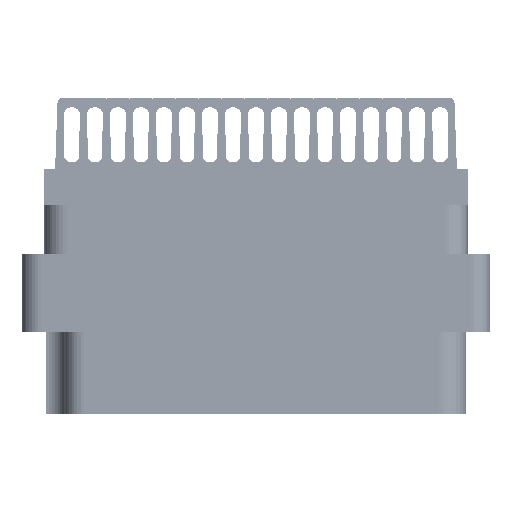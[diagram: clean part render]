
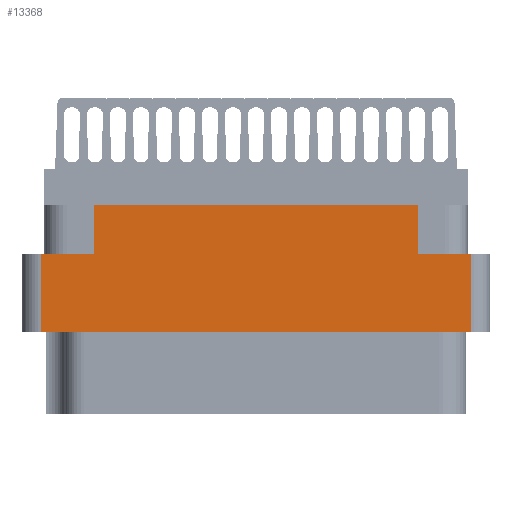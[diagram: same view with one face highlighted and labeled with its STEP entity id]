
A CAD part, left-side view. The second image highlights one B-rep face of the part: STEP entity #13368.
In plain terms, the highlighted planar face has unit normal (-1, 0, 0).
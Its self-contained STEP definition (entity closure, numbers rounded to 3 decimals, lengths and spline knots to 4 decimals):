
#1298 = DIRECTION ( 'NONE',  ( 0., 0., -1. ) ) ;
#3720 = EDGE_CURVE ( 'NONE', #88290, #62367, #60270, .T. ) ;
#4019 = ORIENTED_EDGE ( 'NONE', *, *, #32455, .T. ) ;
#6077 = VECTOR ( 'NONE', #66229, 39.3701 ) ;
#8338 = CARTESIAN_POINT ( 'NONE',  ( -1.375, 0., -0.529 ) ) ;
#9785 = VECTOR ( 'NONE', #70569, 39.3701 ) ;
#10305 = ORIENTED_EDGE ( 'NONE', *, *, #92936, .F. ) ;
#11412 = VERTEX_POINT ( 'NONE', #49687 ) ;
#12026 = VERTEX_POINT ( 'NONE', #71877 ) ;
#12495 = ORIENTED_EDGE ( 'NONE', *, *, #66416, .F. ) ;
#13368 = ADVANCED_FACE ( 'NONE', ( #31602 ), #30020, .T. ) ;
#13901 = VECTOR ( 'NONE', #89599, 39.3701 ) ;
#15624 = DIRECTION ( 'NONE',  ( 0., 1., 0. ) ) ;
#16815 = CARTESIAN_POINT ( 'NONE',  ( -1.375, -0.7005, -0.798 ) ) ;
#18378 = CARTESIAN_POINT ( 'NONE',  ( -1.375, -0.5285, -0.277 ) ) ;
#18799 = VERTEX_POINT ( 'NONE', #53100 ) ;
#23161 = EDGE_LOOP ( 'NONE', ( #43654, #37005, #30594, #29555, #12495, #4019, #10305, #57130 ) ) ;
#26002 = VECTOR ( 'NONE', #35717, 39.3701 ) ;
#26026 = LINE ( 'NONE', #18378, #45294 ) ;
#26498 = CARTESIAN_POINT ( 'NONE',  ( -1.375, 0.5285, -0.277 ) ) ;
#29555 = ORIENTED_EDGE ( 'NONE', *, *, #57769, .T. ) ;
#30020 = PLANE ( 'NONE',  #61913 ) ;
#30327 = CARTESIAN_POINT ( 'NONE',  ( -1.375, 0., -0.277 ) ) ;
#30594 = ORIENTED_EDGE ( 'NONE', *, *, #3720, .F. ) ;
#30751 = CARTESIAN_POINT ( 'NONE',  ( -1.375, 0., -0.277 ) ) ;
#31602 = FACE_OUTER_BOUND ( 'NONE', #23161, .T. ) ;
#32455 = EDGE_CURVE ( 'NONE', #53001, #11412, #26026, .T. ) ;
#34495 = LINE ( 'NONE', #44851, #75499 ) ;
#34787 = CARTESIAN_POINT ( 'NONE',  ( -1.375, 0.7625, -0.117 ) ) ;
#35717 = DIRECTION ( 'NONE',  ( 0., -1., 0. ) ) ;
#37005 = ORIENTED_EDGE ( 'NONE', *, *, #68602, .T. ) ;
#37239 = CARTESIAN_POINT ( 'NONE',  ( -1.375, -0.7625, -0.798 ) ) ;
#37558 = DIRECTION ( 'NONE',  ( -1., 0., 0. ) ) ;
#38107 = VECTOR ( 'NONE', #40411, 39.3701 ) ;
#40411 = DIRECTION ( 'NONE',  ( 0., 0., 1. ) ) ;
#43654 = ORIENTED_EDGE ( 'NONE', *, *, #46906, .F. ) ;
#44851 = CARTESIAN_POINT ( 'NONE',  ( -1.375, 0.7005, -0.798 ) ) ;
#45268 = LINE ( 'NONE', #34787, #26002 ) ;
#45294 = VECTOR ( 'NONE', #84878, 39.3701 ) ;
#46906 = EDGE_CURVE ( 'NONE', #12026, #66844, #60799, .T. ) ;
#48449 = LINE ( 'NONE', #16815, #9785 ) ;
#49687 = CARTESIAN_POINT ( 'NONE',  ( -1.375, -0.5285, -0.117 ) ) ;
#53001 = VERTEX_POINT ( 'NONE', #84582 ) ;
#53100 = CARTESIAN_POINT ( 'NONE',  ( -1.375, 0.5285, -0.117 ) ) ;
#55010 = CARTESIAN_POINT ( 'NONE',  ( -1.375, -0.7005, -0.529 ) ) ;
#57130 = ORIENTED_EDGE ( 'NONE', *, *, #85940, .F. ) ;
#57769 = EDGE_CURVE ( 'NONE', #88290, #93640, #48449, .T. ) ;
#60270 = LINE ( 'NONE', #8338, #73944 ) ;
#60799 = LINE ( 'NONE', #30327, #6077 ) ;
#60881 = LINE ( 'NONE', #26498, #38107 ) ;
#61913 = AXIS2_PLACEMENT_3D ( 'NONE', #37239, #37558, #88225 ) ;
#62367 = VERTEX_POINT ( 'NONE', #72286 ) ;
#66229 = DIRECTION ( 'NONE',  ( 0., -1., 0. ) ) ;
#66416 = EDGE_CURVE ( 'NONE', #53001, #93640, #93603, .T. ) ;
#66844 = VERTEX_POINT ( 'NONE', #87557 ) ;
#68602 = EDGE_CURVE ( 'NONE', #12026, #62367, #34495, .T. ) ;
#70569 = DIRECTION ( 'NONE',  ( 0., 0., 1. ) ) ;
#71877 = CARTESIAN_POINT ( 'NONE',  ( -1.375, 0.7005, -0.277 ) ) ;
#72286 = CARTESIAN_POINT ( 'NONE',  ( -1.375, 0.7005, -0.529 ) ) ;
#73944 = VECTOR ( 'NONE', #15624, 39.3701 ) ;
#75499 = VECTOR ( 'NONE', #1298, 39.3701 ) ;
#84582 = CARTESIAN_POINT ( 'NONE',  ( -1.375, -0.5285, -0.277 ) ) ;
#84878 = DIRECTION ( 'NONE',  ( 0., 0., 1. ) ) ;
#85940 = EDGE_CURVE ( 'NONE', #66844, #18799, #60881, .T. ) ;
#87557 = CARTESIAN_POINT ( 'NONE',  ( -1.375, 0.5285, -0.277 ) ) ;
#88225 = DIRECTION ( 'NONE',  ( 0., 0., 1. ) ) ;
#88290 = VERTEX_POINT ( 'NONE', #55010 ) ;
#89599 = DIRECTION ( 'NONE',  ( 0., -1., 0. ) ) ;
#90740 = CARTESIAN_POINT ( 'NONE',  ( -1.375, -0.7005, -0.277 ) ) ;
#92936 = EDGE_CURVE ( 'NONE', #18799, #11412, #45268, .T. ) ;
#93603 = LINE ( 'NONE', #30751, #13901 ) ;
#93640 = VERTEX_POINT ( 'NONE', #90740 ) ;
